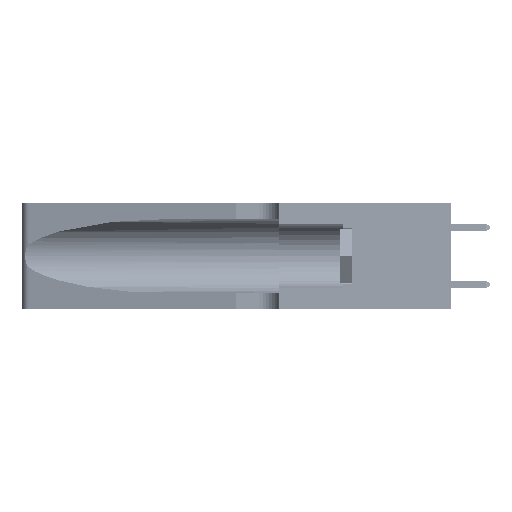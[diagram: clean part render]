
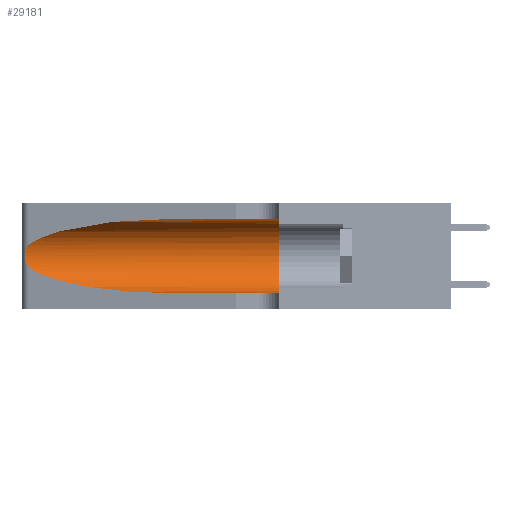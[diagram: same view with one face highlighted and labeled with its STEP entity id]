
A CAD part, left-side view. The second image highlights one B-rep face of the part: STEP entity #29181.
In plain terms, the highlighted cylindrical face has radius 3.308 mm (diameter 6.617 mm), a partial arc.
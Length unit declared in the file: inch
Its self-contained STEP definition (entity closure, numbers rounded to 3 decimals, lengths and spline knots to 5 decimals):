
#198 = ORIENTED_EDGE ( 'NONE', *, *, #5159, .F. ) ;
#1980 = CARTESIAN_POINT ( 'NONE',  ( 0.26018, 1.23835, 0.19895 ) ) ;
#2574 = CARTESIAN_POINT ( 'NONE',  ( 0.1305, 0.72297, 0.05475 ) ) ;
#4104 = ORIENTED_EDGE ( 'NONE', *, *, #31438, .F. ) ;
#4822 = DIRECTION ( 'NONE',  ( 0., -1., 0. ) ) ;
#5101 = VECTOR ( 'NONE', #53326, 39.37008 ) ;
#5159 = EDGE_CURVE ( 'NONE', #28196, #24125, #24656, .T. ) ;
#6247 = CARTESIAN_POINT ( 'NONE',  ( 0.26075, 1.23896, 0.178 ) ) ;
#7258 = CARTESIAN_POINT ( 'NONE',  ( 0.18966, 0.96281, 0.05475 ) ) ;
#7383 = LINE ( 'NONE', #34367, #28785 ) ;
#8874 = DIRECTION ( 'NONE',  ( 0., -1., 0. ) ) ;
#10335 = CARTESIAN_POINT ( 'NONE',  ( 0.25555, 1.22994, 0.2215 ) ) ;
#10524 = CARTESIAN_POINT ( 'NONE',  ( 0.25856, 1.23593, 0.16098 ) ) ;
#10557 = CARTESIAN_POINT ( 'NONE',  ( 0.1305, 0.72297, 0.31525 ) ) ;
#10845 = ORIENTED_EDGE ( 'NONE', *, *, #54597, .T. ) ;
#10879 = FACE_OUTER_BOUND ( 'NONE', #53832, .T. ) ;
#11643 = CARTESIAN_POINT ( 'NONE',  ( 0.1305, 0.35, 0.31525 ) ) ;
#13414 = ORIENTED_EDGE ( 'NONE', *, *, #24050, .T. ) ;
#13711 = DIRECTION ( 'NONE',  ( 0., 1., 0. ) ) ;
#14574 = ORIENTED_EDGE ( 'NONE', *, *, #43375, .T. ) ;
#14782 = CARTESIAN_POINT ( 'NONE',  ( 0.25639, 1.23186, 0.15144 ) ) ;
#14809 = CARTESIAN_POINT ( 'NONE',  ( 0.18966, 0.96281, 0.31525 ) ) ;
#15159 = AXIS2_PLACEMENT_3D ( 'NONE', #39101, #13711, #43293 ) ;
#16954 = CARTESIAN_POINT ( 'NONE',  ( 0.1305, 0.35, 0.05475 ) ) ;
#19128 = CARTESIAN_POINT ( 'NONE',  ( 0.25487, 1.22718, 0.14631 ) ) ;
#19158 = CARTESIAN_POINT ( 'NONE',  ( 0.25487, 1.22718, 0.22369 ) ) ;
#19744 = CARTESIAN_POINT ( 'NONE',  ( 0.1305, 1.61858, 0.05475 ) ) ;
#23226 = CARTESIAN_POINT ( 'NONE',  ( 0.25639, 1.23184, 0.21858 ) ) ;
#23944 = B_SPLINE_CURVE_WITH_KNOTS ( 'NONE', 3,
 ( #39976, #10335, #23226, #52541, #27559, #1980, #31767, #6247, #35973, #10524, #40148, #14782, #44371, #19128 ),
 .UNSPECIFIED., .F., .F.,
 ( 4, 2, 2, 2, 2, 2, 4 ),
 ( 0., 0.00027, 0.00053, 0.00107, 0.0016, 0.00187, 0.00214 ),
 .UNSPECIFIED. ) ;
#24050 = EDGE_CURVE ( 'NONE', #26044, #27485, #28093, .T. ) ;
#24125 = VERTEX_POINT ( 'NONE', #16954 ) ;
#24428 = CARTESIAN_POINT ( 'NONE',  ( 0.1305, 0.72297, 0.05475 ) ) ;
#24656 = CIRCLE ( 'NONE', #15159, 0.13025 ) ;
#26044 = VERTEX_POINT ( 'NONE', #45737 ) ;
#26105 = CARTESIAN_POINT ( 'NONE',  ( 0.1305, 1.61858, 0.185 ) ) ;
#27485 = VERTEX_POINT ( 'NONE', #2574 ) ;
#27559 = CARTESIAN_POINT ( 'NONE',  ( 0.25854, 1.2359, 0.20912 ) ) ;
#28093 =( BOUNDED_CURVE ( )  B_SPLINE_CURVE ( 3, ( #49551, #41139, #7258, #24428 ),
 .UNSPECIFIED., .F., .F. ) 
 B_SPLINE_CURVE_WITH_KNOTS ( ( 4, 4 ),
 ( 3.44316, 4.71239 ),
 .UNSPECIFIED. ) 
 CURVE ( )  GEOMETRIC_REPRESENTATION_ITEM ( )  RATIONAL_B_SPLINE_CURVE ( ( 1., 0.87, 0.87, 1. ) ) 
 REPRESENTATION_ITEM ( '' )  );
#28196 = VERTEX_POINT ( 'NONE', #11643 ) ;
#28785 = VECTOR ( 'NONE', #8874, 39.37008 ) ;
#29181 = ADVANCED_FACE ( 'NONE', ( #10879 ), #43312, .F. ) ;
#29597 = VERTEX_POINT ( 'NONE', #43648 ) ;
#30359 = DIRECTION ( 'NONE',  ( 0., 0., -1. ) ) ;
#31438 = EDGE_CURVE ( 'NONE', #29597, #28196, #7383, .T. ) ;
#31767 = CARTESIAN_POINT ( 'NONE',  ( 0.26075, 1.23896, 0.19203 ) ) ;
#34367 = CARTESIAN_POINT ( 'NONE',  ( 0.1305, 1.61858, 0.31525 ) ) ;
#34651 = ORIENTED_EDGE ( 'NONE', *, *, #46726, .T. ) ;
#35973 = CARTESIAN_POINT ( 'NONE',  ( 0.26017, 1.23833, 0.17102 ) ) ;
#39101 = CARTESIAN_POINT ( 'NONE',  ( 0.1305, 0.35, 0.185 ) ) ;
#39976 = CARTESIAN_POINT ( 'NONE',  ( 0.25487, 1.22718, 0.22369 ) ) ;
#40148 = CARTESIAN_POINT ( 'NONE',  ( 0.25789, 1.23486, 0.15765 ) ) ;
#41139 = CARTESIAN_POINT ( 'NONE',  ( 0.2373, 1.15595, 0.08982 ) ) ;
#43293 = DIRECTION ( 'NONE',  ( 0., 0., 1. ) ) ;
#43312 = CYLINDRICAL_SURFACE ( 'NONE', #44544, 0.13025 ) ;
#43375 = EDGE_CURVE ( 'NONE', #44784, #26044, #23944, .T. ) ;
#43648 = CARTESIAN_POINT ( 'NONE',  ( 0.1305, 0.72297, 0.31525 ) ) ;
#44371 = CARTESIAN_POINT ( 'NONE',  ( 0.25555, 1.22993, 0.14849 ) ) ;
#44396 = CARTESIAN_POINT ( 'NONE',  ( 0.2373, 1.15595, 0.28018 ) ) ;
#44544 = AXIS2_PLACEMENT_3D ( 'NONE', #26105, #4822, #30359 ) ;
#44784 = VERTEX_POINT ( 'NONE', #45729 ) ;
#45729 = CARTESIAN_POINT ( 'NONE',  ( 0.25487, 1.22718, 0.22369 ) ) ;
#45737 = CARTESIAN_POINT ( 'NONE',  ( 0.25487, 1.22718, 0.14631 ) ) ;
#46726 = EDGE_CURVE ( 'NONE', #27485, #24125, #50059, .T. ) ;
#49177 =( BOUNDED_CURVE ( )  B_SPLINE_CURVE ( 3, ( #10557, #14809, #44396, #19158 ),
 .UNSPECIFIED., .F., .T. ) 
 B_SPLINE_CURVE_WITH_KNOTS ( ( 4, 4 ),
 ( 1.5708, 2.84003 ),
 .UNSPECIFIED. ) 
 CURVE ( )  GEOMETRIC_REPRESENTATION_ITEM ( )  RATIONAL_B_SPLINE_CURVE ( ( 1., 0.87, 0.87, 1. ) ) 
 REPRESENTATION_ITEM ( '' )  );
#49551 = CARTESIAN_POINT ( 'NONE',  ( 0.25487, 1.22718, 0.14631 ) ) ;
#50059 = LINE ( 'NONE', #19744, #5101 ) ;
#52541 = CARTESIAN_POINT ( 'NONE',  ( 0.25787, 1.23484, 0.2124 ) ) ;
#53326 = DIRECTION ( 'NONE',  ( 0., -1., 0. ) ) ;
#53832 = EDGE_LOOP ( 'NONE', ( #10845, #14574, #13414, #34651, #198, #4104 ) ) ;
#54597 = EDGE_CURVE ( 'NONE', #29597, #44784, #49177, .T. ) ;
